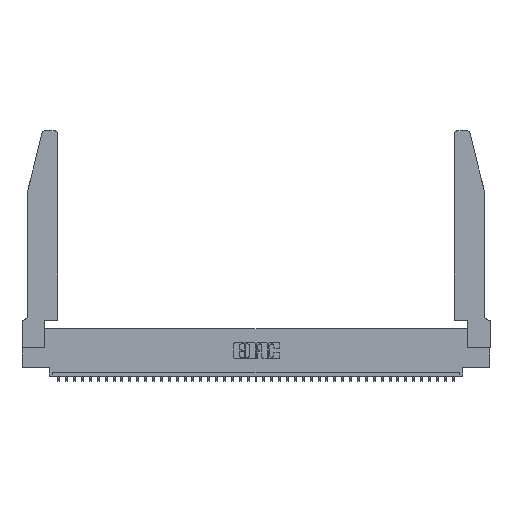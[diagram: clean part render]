
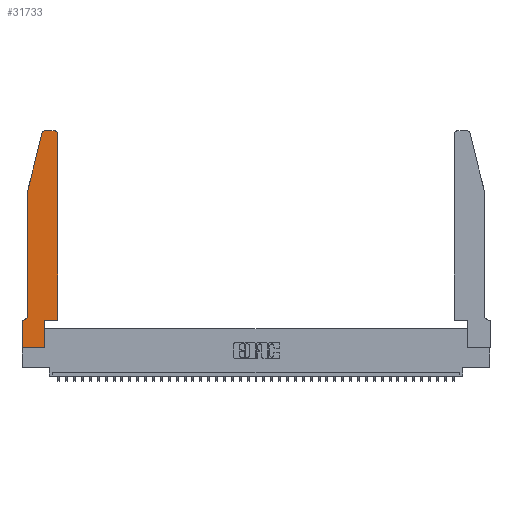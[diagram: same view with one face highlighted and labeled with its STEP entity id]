
A CAD part, top view. The second image highlights one B-rep face of the part: STEP entity #31733.
In plain terms, the highlighted planar face has unit normal (0, 0, 1).
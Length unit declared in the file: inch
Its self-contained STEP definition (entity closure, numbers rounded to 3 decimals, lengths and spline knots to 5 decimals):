
#353 = DIRECTION ( 'NONE',  ( 0., 0., -1. ) ) ;
#984 = LINE ( 'NONE', #30983, #25935 ) ;
#1354 = DIRECTION ( 'NONE',  ( 0., 1., 0. ) ) ;
#1677 = DIRECTION ( 'NONE',  ( 0., -1., 0. ) ) ;
#1808 = EDGE_LOOP ( 'NONE', ( #16994, #15037, #12477, #19044, #33241, #32198, #39003, #29568, #22674, #30574, #11325, #6914 ) ) ;
#2063 = AXIS2_PLACEMENT_3D ( 'NONE', #38627, #41877, #2657 ) ;
#2175 = VECTOR ( 'NONE', #30763, 39.37008 ) ;
#2221 = CARTESIAN_POINT ( 'NONE',  ( 0.2865, 0., 0.37 ) ) ;
#2233 = DIRECTION ( 'NONE',  ( 0., 1., 0. ) ) ;
#2345 = VECTOR ( 'NONE', #36469, 39.37008 ) ;
#2600 = CARTESIAN_POINT ( 'NONE',  ( 0.2605, 2.75, 0.37 ) ) ;
#2657 = DIRECTION ( 'NONE',  ( 1., 0., 0. ) ) ;
#2868 = VERTEX_POINT ( 'NONE', #13197 ) ;
#3798 = VERTEX_POINT ( 'NONE', #22823 ) ;
#4090 = DIRECTION ( 'NONE',  ( 0., 0., 1. ) ) ;
#4464 = CARTESIAN_POINT ( 'NONE',  ( 0.284, 2.75, 0.37 ) ) ;
#5216 = LINE ( 'NONE', #20644, #2175 ) ;
#5506 = CARTESIAN_POINT ( 'NONE',  ( 0.4505, 2.72, 0.37 ) ) ;
#5706 = VERTEX_POINT ( 'NONE', #35789 ) ;
#5765 = DIRECTION ( 'NONE',  ( 1., 0., 0. ) ) ;
#6487 = EDGE_CURVE ( 'NONE', #3798, #5706, #41646, .T. ) ;
#6631 = DIRECTION ( 'NONE',  ( -1., 0., 0. ) ) ;
#6914 = ORIENTED_EDGE ( 'NONE', *, *, #36196, .T. ) ;
#7315 = CARTESIAN_POINT ( 'NONE',  ( 0.0755, 0.35, 0.37 ) ) ;
#9627 = EDGE_CURVE ( 'NONE', #12689, #31092, #40890, .T. ) ;
#10110 = LINE ( 'NONE', #2600, #36599 ) ;
#10133 = VECTOR ( 'NONE', #2233, 39.37008 ) ;
#10562 = CARTESIAN_POINT ( 'NONE',  ( 0.0055, 0.35, 0.37 ) ) ;
#11325 = ORIENTED_EDGE ( 'NONE', *, *, #20991, .T. ) ;
#12180 = VECTOR ( 'NONE', #1677, 39.37008 ) ;
#12337 = CARTESIAN_POINT ( 'NONE',  ( 0.25487, 2.72718, 0.37 ) ) ;
#12477 = ORIENTED_EDGE ( 'NONE', *, *, #40274, .T. ) ;
#12487 = CARTESIAN_POINT ( 'NONE',  ( 0.4505, 0.35, 0.37 ) ) ;
#12689 = VERTEX_POINT ( 'NONE', #37016 ) ;
#13197 = CARTESIAN_POINT ( 'NONE',  ( 0.4205, 2.75, 0.37 ) ) ;
#13400 = CIRCLE ( 'NONE', #32320, 0.07 ) ;
#13683 = CARTESIAN_POINT ( 'NONE',  ( 0., 0.35, 0.37 ) ) ;
#13992 = CARTESIAN_POINT ( 'NONE',  ( 0., 0., 0.37 ) ) ;
#14023 = EDGE_CURVE ( 'NONE', #2868, #21156, #10110, .T. ) ;
#15037 = ORIENTED_EDGE ( 'NONE', *, *, #41850, .T. ) ;
#15378 = LINE ( 'NONE', #21126, #21943 ) ;
#15565 = EDGE_CURVE ( 'NONE', #23975, #12689, #38985, .T. ) ;
#16278 = AXIS2_PLACEMENT_3D ( 'NONE', #13683, #4090, #36400 ) ;
#16994 = ORIENTED_EDGE ( 'NONE', *, *, #14023, .T. ) ;
#17205 = AXIS2_PLACEMENT_3D ( 'NONE', #35637, #25419, #5765 ) ;
#18127 = DIRECTION ( 'NONE',  ( -0.239, -0.971, 0. ) ) ;
#19044 = ORIENTED_EDGE ( 'NONE', *, *, #6487, .T. ) ;
#19173 = DIRECTION ( 'NONE',  ( 0., -1., 0. ) ) ;
#20644 = CARTESIAN_POINT ( 'NONE',  ( 0.4505, 0.35, 0.37 ) ) ;
#20702 = CARTESIAN_POINT ( 'NONE',  ( 0.2865, 0.35, 0.37 ) ) ;
#20795 = EDGE_CURVE ( 'NONE', #31092, #34597, #984, .T. ) ;
#20840 = CIRCLE ( 'NONE', #17205, 0.03 ) ;
#20991 = EDGE_CURVE ( 'NONE', #26675, #28857, #22339, .T. ) ;
#21126 = CARTESIAN_POINT ( 'NONE',  ( 0.0755, 2., 0.37 ) ) ;
#21156 = VERTEX_POINT ( 'NONE', #4464 ) ;
#21378 = DIRECTION ( 'NONE',  ( -1., 0., 0. ) ) ;
#21943 = VECTOR ( 'NONE', #18127, 39.37008 ) ;
#22217 = CARTESIAN_POINT ( 'NONE',  ( 0.4505, 0.35, 0.37 ) ) ;
#22339 = LINE ( 'NONE', #12487, #10133 ) ;
#22674 = ORIENTED_EDGE ( 'NONE', *, *, #27299, .T. ) ;
#22823 = CARTESIAN_POINT ( 'NONE',  ( 0.0755, 2., 0.37 ) ) ;
#22982 = VERTEX_POINT ( 'NONE', #39923 ) ;
#23729 = PLANE ( 'NONE',  #16278 ) ;
#23975 = VERTEX_POINT ( 'NONE', #10562 ) ;
#24209 = EDGE_CURVE ( 'NONE', #22982, #26675, #5216, .T. ) ;
#24846 = VECTOR ( 'NONE', #1354, 39.37008 ) ;
#25419 = DIRECTION ( 'NONE',  ( 0., 0., 1. ) ) ;
#25935 = VECTOR ( 'NONE', #40349, 39.37008 ) ;
#25976 = VERTEX_POINT ( 'NONE', #12337 ) ;
#26130 = CARTESIAN_POINT ( 'NONE',  ( 0.0055, 0.42, 0.37 ) ) ;
#26675 = VERTEX_POINT ( 'NONE', #22217 ) ;
#27299 = EDGE_CURVE ( 'NONE', #34597, #22982, #37571, .T. ) ;
#28358 = CIRCLE ( 'NONE', #2063, 0.03 ) ;
#28857 = VERTEX_POINT ( 'NONE', #5506 ) ;
#29568 = ORIENTED_EDGE ( 'NONE', *, *, #20795, .T. ) ;
#30208 = FACE_OUTER_BOUND ( 'NONE', #1808, .T. ) ;
#30574 = ORIENTED_EDGE ( 'NONE', *, *, #24209, .T. ) ;
#30763 = DIRECTION ( 'NONE',  ( 1., 0., 0. ) ) ;
#30983 = CARTESIAN_POINT ( 'NONE',  ( 0., 0., 0.37 ) ) ;
#31092 = VERTEX_POINT ( 'NONE', #13992 ) ;
#31733 = ADVANCED_FACE ( 'NONE', ( #30208 ), #23729, .T. ) ;
#31818 = CARTESIAN_POINT ( 'NONE',  ( 0., 0., 0.37 ) ) ;
#32162 = EDGE_CURVE ( 'NONE', #5706, #23975, #13400, .T. ) ;
#32198 = ORIENTED_EDGE ( 'NONE', *, *, #15565, .T. ) ;
#32320 = AXIS2_PLACEMENT_3D ( 'NONE', #26130, #353, #6631 ) ;
#33241 = ORIENTED_EDGE ( 'NONE', *, *, #32162, .T. ) ;
#34597 = VERTEX_POINT ( 'NONE', #2221 ) ;
#35637 = CARTESIAN_POINT ( 'NONE',  ( 0.4205, 2.72, 0.37 ) ) ;
#35789 = CARTESIAN_POINT ( 'NONE',  ( 0.0755, 0.42, 0.37 ) ) ;
#36196 = EDGE_CURVE ( 'NONE', #28857, #2868, #20840, .T. ) ;
#36400 = DIRECTION ( 'NONE',  ( 1., 0., 0. ) ) ;
#36469 = DIRECTION ( 'NONE',  ( -1., 0., 0. ) ) ;
#36599 = VECTOR ( 'NONE', #21378, 39.37008 ) ;
#37016 = CARTESIAN_POINT ( 'NONE',  ( 0., 0.35, 0.37 ) ) ;
#37240 = CARTESIAN_POINT ( 'NONE',  ( 0.0755, 2., 0.37 ) ) ;
#37571 = LINE ( 'NONE', #20702, #24846 ) ;
#37848 = VECTOR ( 'NONE', #19173, 39.37008 ) ;
#38627 = CARTESIAN_POINT ( 'NONE',  ( 0.284, 2.72, 0.37 ) ) ;
#38985 = LINE ( 'NONE', #7315, #2345 ) ;
#39003 = ORIENTED_EDGE ( 'NONE', *, *, #9627, .T. ) ;
#39923 = CARTESIAN_POINT ( 'NONE',  ( 0.2865, 0.35, 0.37 ) ) ;
#40274 = EDGE_CURVE ( 'NONE', #25976, #3798, #15378, .T. ) ;
#40349 = DIRECTION ( 'NONE',  ( 1., 0., 0. ) ) ;
#40890 = LINE ( 'NONE', #31818, #37848 ) ;
#41646 = LINE ( 'NONE', #37240, #12180 ) ;
#41850 = EDGE_CURVE ( 'NONE', #21156, #25976, #28358, .T. ) ;
#41877 = DIRECTION ( 'NONE',  ( 0., 0., 1. ) ) ;
